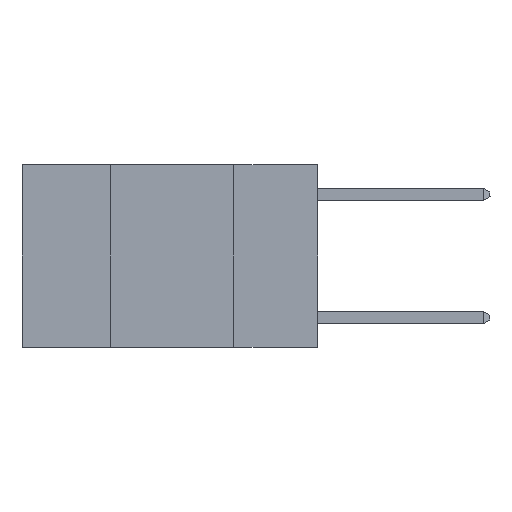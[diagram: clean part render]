
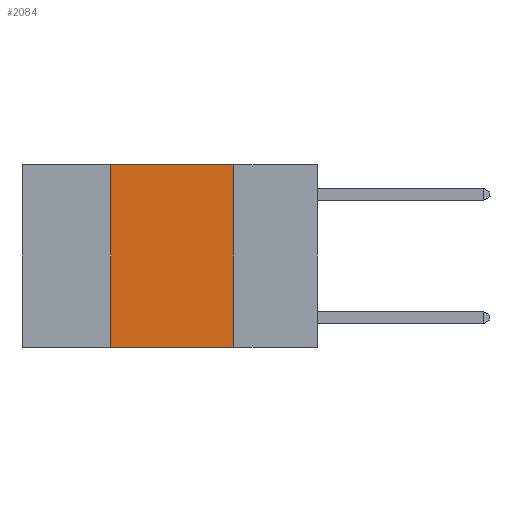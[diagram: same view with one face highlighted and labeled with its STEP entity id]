
A CAD part, left-side view. The second image highlights one B-rep face of the part: STEP entity #2084.
In plain terms, the highlighted planar face has unit normal (-1, 0, 0).
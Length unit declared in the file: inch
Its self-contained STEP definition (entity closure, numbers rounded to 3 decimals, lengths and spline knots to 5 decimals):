
#2084 = ADVANCED_FACE ( 'NONE', ( #7258 ), #15426, .F. ) ;
#2495 = EDGE_LOOP ( 'NONE', ( #15708, #7451, #8206, #12109 ) ) ;
#3218 = CARTESIAN_POINT ( 'NONE',  ( 0., 0.17, 0. ) ) ;
#3259 = VECTOR ( 'NONE', #16099, 39.37008 ) ;
#3455 = EDGE_CURVE ( 'NONE', #14870, #8871, #15973, .T. ) ;
#3523 = CARTESIAN_POINT ( 'NONE',  ( 0., 0.42, 0. ) ) ;
#3765 = CARTESIAN_POINT ( 'NONE',  ( 0., 0.42, -0.37 ) ) ;
#4046 = DIRECTION ( 'NONE',  ( 0., -1., 0. ) ) ;
#4532 = CARTESIAN_POINT ( 'NONE',  ( 0., 0.6, 0. ) ) ;
#7258 = FACE_OUTER_BOUND ( 'NONE', #2495, .T. ) ;
#7307 = DIRECTION ( 'NONE',  ( 0., 0., -1. ) ) ;
#7379 = VECTOR ( 'NONE', #7307, 39.37008 ) ;
#7451 = ORIENTED_EDGE ( 'NONE', *, *, #15859, .F. ) ;
#7471 = VECTOR ( 'NONE', #14673, 39.37008 ) ;
#8206 = ORIENTED_EDGE ( 'NONE', *, *, #3455, .F. ) ;
#8643 = LINE ( 'NONE', #3218, #7379 ) ;
#8871 = VERTEX_POINT ( 'NONE', #17004 ) ;
#9164 = LINE ( 'NONE', #13331, #3259 ) ;
#9205 = LINE ( 'NONE', #13543, #14982 ) ;
#11519 = CARTESIAN_POINT ( 'NONE',  ( 0., 0.17, 0. ) ) ;
#11728 = EDGE_CURVE ( 'NONE', #14870, #15869, #9164, .T. ) ;
#12109 = ORIENTED_EDGE ( 'NONE', *, *, #11728, .T. ) ;
#12350 = CARTESIAN_POINT ( 'NONE',  ( 0., 0.17, -0.37 ) ) ;
#12657 = DIRECTION ( 'NONE',  ( 0., 0., -1. ) ) ;
#12949 = DIRECTION ( 'NONE',  ( 1., 0., 0. ) ) ;
#13331 = CARTESIAN_POINT ( 'NONE',  ( 0., 0.6, -0.37 ) ) ;
#13428 = VERTEX_POINT ( 'NONE', #11519 ) ;
#13543 = CARTESIAN_POINT ( 'NONE',  ( 0., 0.6, 0. ) ) ;
#13910 = AXIS2_PLACEMENT_3D ( 'NONE', #4532, #12949, #12657 ) ;
#14673 = DIRECTION ( 'NONE',  ( 0., 0., 1. ) ) ;
#14835 = EDGE_CURVE ( 'NONE', #13428, #15869, #8643, .T. ) ;
#14870 = VERTEX_POINT ( 'NONE', #3765 ) ;
#14982 = VECTOR ( 'NONE', #4046, 39.37008 ) ;
#15426 = PLANE ( 'NONE',  #13910 ) ;
#15708 = ORIENTED_EDGE ( 'NONE', *, *, #14835, .F. ) ;
#15859 = EDGE_CURVE ( 'NONE', #8871, #13428, #9205, .T. ) ;
#15869 = VERTEX_POINT ( 'NONE', #12350 ) ;
#15973 = LINE ( 'NONE', #3523, #7471 ) ;
#16099 = DIRECTION ( 'NONE',  ( 0., -1., 0. ) ) ;
#17004 = CARTESIAN_POINT ( 'NONE',  ( 0., 0.42, 0. ) ) ;
